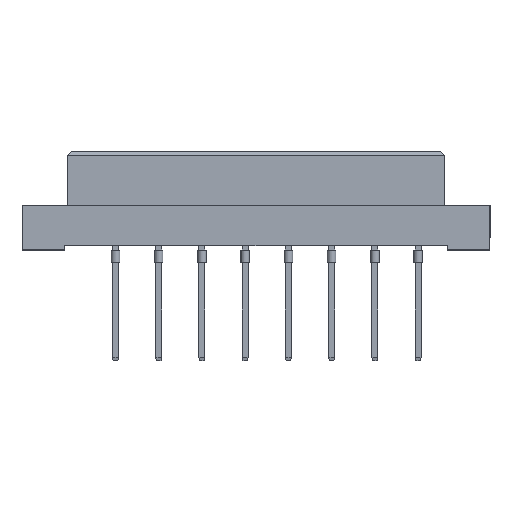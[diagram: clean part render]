
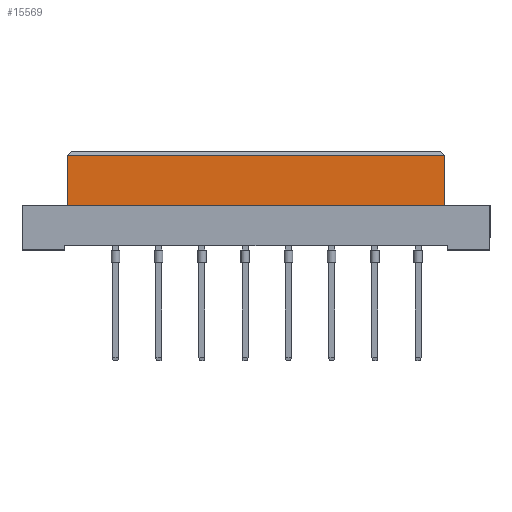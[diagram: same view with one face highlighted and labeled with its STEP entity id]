
A CAD part, top view. The second image highlights one B-rep face of the part: STEP entity #15569.
In plain terms, the highlighted planar face has unit normal (0, 0, 1).
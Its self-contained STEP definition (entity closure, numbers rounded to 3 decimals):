
#203 = ORIENTED_EDGE ( 'NONE', *, *, #2033, .T. ) ;
#1402 = EDGE_CURVE ( 'NONE', #12707, #20272, #7445, .T. ) ;
#2033 = EDGE_CURVE ( 'NONE', #12707, #5734, #11335, .T. ) ;
#2164 = DIRECTION ( 'NONE',  ( 1., 0., 0. ) ) ;
#2318 = VERTEX_POINT ( 'NONE', #19197 ) ;
#3423 = CARTESIAN_POINT ( 'NONE',  ( 22.2, -6.4, 4.25 ) ) ;
#4393 = ORIENTED_EDGE ( 'NONE', *, *, #13707, .T. ) ;
#5127 = CARTESIAN_POINT ( 'NONE',  ( 22.2, -6.4, 4.25 ) ) ;
#5234 = DIRECTION ( 'NONE',  ( 0., 1., 0. ) ) ;
#5453 = CARTESIAN_POINT ( 'NONE',  ( -22.2, -0.5, 4.25 ) ) ;
#5734 = VERTEX_POINT ( 'NONE', #18566 ) ;
#5884 = DIRECTION ( 'NONE',  ( 0., 1., 0. ) ) ;
#6502 = VECTOR ( 'NONE', #5234, 1000. ) ;
#6805 = DIRECTION ( 'NONE',  ( -1., 0., 0. ) ) ;
#6876 = EDGE_CURVE ( 'NONE', #2318, #20272, #11773, .T. ) ;
#7221 = PLANE ( 'NONE',  #20282 ) ;
#7445 = LINE ( 'NONE', #12403, #11608 ) ;
#7904 = CARTESIAN_POINT ( 'NONE',  ( -22.2, -0.5, 4.25 ) ) ;
#8288 = EDGE_LOOP ( 'NONE', ( #4393, #15169, #19787, #203 ) ) ;
#8792 = DIRECTION ( 'NONE',  ( 1., 0., 0. ) ) ;
#11335 = LINE ( 'NONE', #3423, #12232 ) ;
#11608 = VECTOR ( 'NONE', #5884, 1000. ) ;
#11773 = LINE ( 'NONE', #5453, #18288 ) ;
#11974 = CARTESIAN_POINT ( 'NONE',  ( 22.2, -6.4, 4.25 ) ) ;
#12232 = VECTOR ( 'NONE', #2164, 1000. ) ;
#12388 = CARTESIAN_POINT ( 'NONE',  ( -22.2, -6.4, 4.25 ) ) ;
#12403 = CARTESIAN_POINT ( 'NONE',  ( -22.2, -6.4, 4.25 ) ) ;
#12707 = VERTEX_POINT ( 'NONE', #12388 ) ;
#13135 = LINE ( 'NONE', #5127, #6502 ) ;
#13707 = EDGE_CURVE ( 'NONE', #5734, #2318, #13135, .T. ) ;
#15001 = FACE_OUTER_BOUND ( 'NONE', #8288, .T. ) ;
#15169 = ORIENTED_EDGE ( 'NONE', *, *, #6876, .T. ) ;
#15569 = ADVANCED_FACE ( 'NONE', ( #15001 ), #7221, .T. ) ;
#18288 = VECTOR ( 'NONE', #6805, 1000. ) ;
#18366 = DIRECTION ( 'NONE',  ( 0., 0., 1. ) ) ;
#18566 = CARTESIAN_POINT ( 'NONE',  ( 22.2, -6.4, 4.25 ) ) ;
#19197 = CARTESIAN_POINT ( 'NONE',  ( 22.2, -0.5, 4.25 ) ) ;
#19787 = ORIENTED_EDGE ( 'NONE', *, *, #1402, .F. ) ;
#20272 = VERTEX_POINT ( 'NONE', #7904 ) ;
#20282 = AXIS2_PLACEMENT_3D ( 'NONE', #11974, #18366, #8792 ) ;
